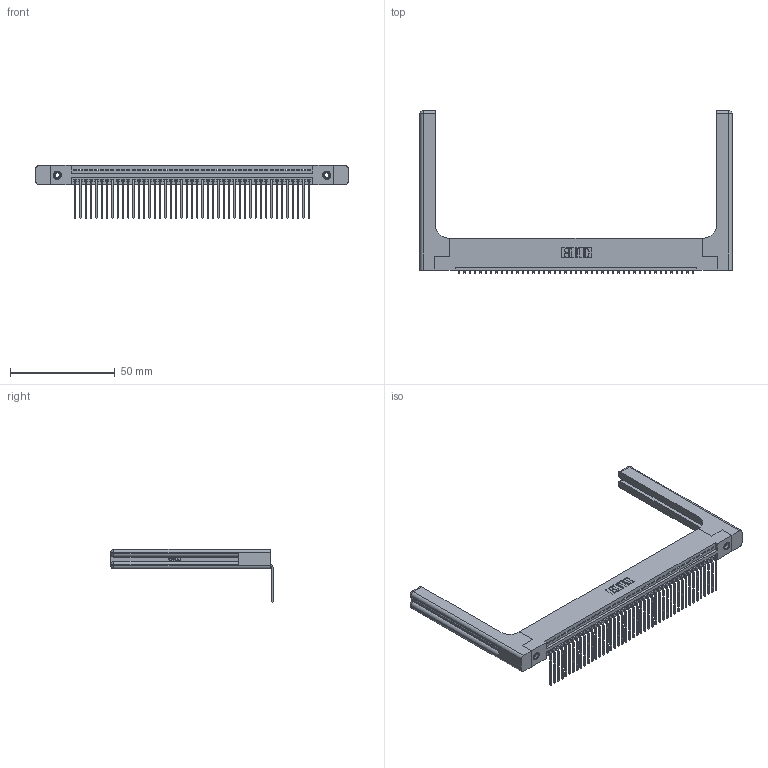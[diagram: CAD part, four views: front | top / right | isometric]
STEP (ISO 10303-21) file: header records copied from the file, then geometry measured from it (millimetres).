
FILE_DESCRIPTION (( 'STEP AP203' ), '1' );
FILE_NAME ('395-045-559-158.STEP', '2019-10-22T19:40:19', ( '' ), ( '' ), 'SwSTEP 2.0', 'SolidWorks 2016', '' );
FILE_SCHEMA (( 'CONFIG_CONTROL_DESIGN' ));
Length unit declared in the file: inch
Products named in the file (5): 345-292-001_558 559 Tail - 1; 345-250-001_345-250-001-102; 345-220-058_345-220-058; 345 Part_Flush Mounting Lugs - 0.156 Dia-TH; 395-045-559-158
Assembly tree (50 placements, depth 2):
  395-045-559-158
    345 Part_Flush Mounting Lugs - 0.156 Dia-TH
    345-292-001_558 559 Tail - 1  x45
    345-250-001_345-250-001-102  x2
    345-220-058_345-220-058  x2
Bounding box: 149.33 x 77.71 x 25.53 mm (x, y, z)
Volume: 22862.7 mm3; surface area: 25307.4 mm2
Topology: 50 solids, 50 shells, 3082 faces, 9197 edges, 6050 vertices
Faces by surface type: plane 2118, cylinder 904, bspline 36, cone 12, sphere 8, torus 4
Entity records: 38730 total; most frequent: CARTESIAN_POINT 7680, ORIENTED_EDGE 6456, DIRECTION 5650, EDGE_CURVE 3228, VECTOR 2824, LINE 2824, VERTEX_POINT 2142, AXIS2_PLACEMENT_3D 1413
